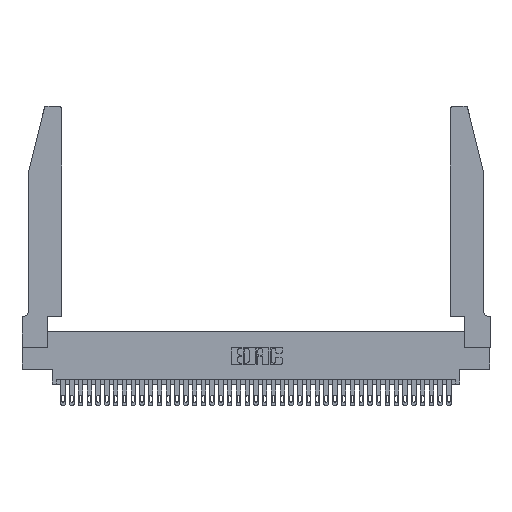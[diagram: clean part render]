
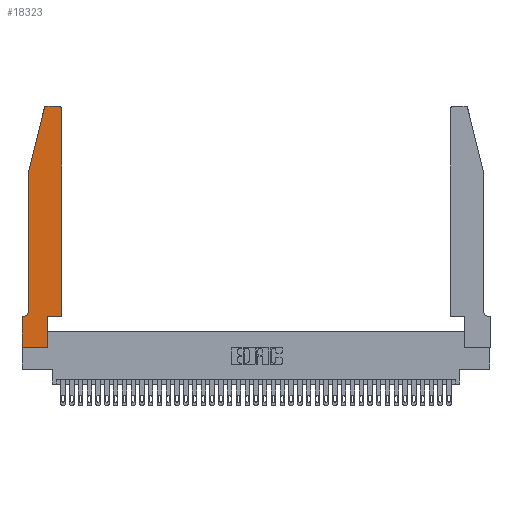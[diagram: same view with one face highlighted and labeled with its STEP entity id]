
A CAD part, top view. The second image highlights one B-rep face of the part: STEP entity #18323.
In plain terms, the highlighted planar face has unit normal (0, 0, 1).
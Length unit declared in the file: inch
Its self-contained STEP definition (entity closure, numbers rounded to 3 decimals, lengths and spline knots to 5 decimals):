
#86 = VERTEX_POINT ( 'NONE', #29668 ) ;
#151 = EDGE_CURVE ( 'NONE', #86, #35048, #34233, .T. ) ;
#384 = CARTESIAN_POINT ( 'NONE',  ( 0.0055, 0.42, 0.37 ) ) ;
#791 = ORIENTED_EDGE ( 'NONE', *, *, #26807, .T. ) ;
#1087 = EDGE_CURVE ( 'NONE', #15926, #29225, #2932, .T. ) ;
#1210 = ORIENTED_EDGE ( 'NONE', *, *, #21746, .T. ) ;
#1305 = DIRECTION ( 'NONE',  ( 1., 0., 0. ) ) ;
#2008 = CARTESIAN_POINT ( 'NONE',  ( 0.4505, 0.35, 0.37 ) ) ;
#2932 = LINE ( 'NONE', #17057, #21660 ) ;
#3139 = CARTESIAN_POINT ( 'NONE',  ( 0.2865, 0.35, 0.37 ) ) ;
#3264 = DIRECTION ( 'NONE',  ( 0., 1., 0. ) ) ;
#3406 = AXIS2_PLACEMENT_3D ( 'NONE', #35109, #4677, #38346 ) ;
#3493 = DIRECTION ( 'NONE',  ( 0., 0., -1. ) ) ;
#3570 = EDGE_CURVE ( 'NONE', #39554, #4459, #31378, .T. ) ;
#3728 = LINE ( 'NONE', #16018, #23432 ) ;
#3960 = ORIENTED_EDGE ( 'NONE', *, *, #21685, .T. ) ;
#4459 = VERTEX_POINT ( 'NONE', #37894 ) ;
#4586 = LINE ( 'NONE', #4966, #18542 ) ;
#4677 = DIRECTION ( 'NONE',  ( 0., 0., 1. ) ) ;
#4966 = CARTESIAN_POINT ( 'NONE',  ( 0., 0., 0.37 ) ) ;
#5246 = DIRECTION ( 'NONE',  ( -1., 0., 0. ) ) ;
#5284 = FACE_OUTER_BOUND ( 'NONE', #33183, .T. ) ;
#6537 = CARTESIAN_POINT ( 'NONE',  ( 0.0755, 0.42, 0.37 ) ) ;
#6699 = DIRECTION ( 'NONE',  ( 0., 1., 0. ) ) ;
#7874 = VERTEX_POINT ( 'NONE', #13865 ) ;
#8078 = VECTOR ( 'NONE', #21347, 39.37008 ) ;
#13363 = DIRECTION ( 'NONE',  ( 0., 0., 1. ) ) ;
#13376 = DIRECTION ( 'NONE',  ( 0., 0., 1. ) ) ;
#13865 = CARTESIAN_POINT ( 'NONE',  ( 0.4205, 2.75, 0.37 ) ) ;
#14188 = CARTESIAN_POINT ( 'NONE',  ( 0.2865, 0.35, 0.37 ) ) ;
#14258 = AXIS2_PLACEMENT_3D ( 'NONE', #34974, #13376, #38065 ) ;
#14449 = CARTESIAN_POINT ( 'NONE',  ( 0.4505, 2.72, 0.37 ) ) ;
#15034 = CARTESIAN_POINT ( 'NONE',  ( 0.0755, 2., 0.37 ) ) ;
#15319 = EDGE_CURVE ( 'NONE', #7874, #36643, #25417, .T. ) ;
#15326 = CARTESIAN_POINT ( 'NONE',  ( 0.0755, 2., 0.37 ) ) ;
#15926 = VERTEX_POINT ( 'NONE', #21176 ) ;
#16018 = CARTESIAN_POINT ( 'NONE',  ( 0.4505, 0.35, 0.37 ) ) ;
#16078 = VECTOR ( 'NONE', #27259, 39.37008 ) ;
#16306 = VECTOR ( 'NONE', #5246, 39.37008 ) ;
#16720 = ORIENTED_EDGE ( 'NONE', *, *, #38803, .T. ) ;
#17057 = CARTESIAN_POINT ( 'NONE',  ( 0., 0., 0.37 ) ) ;
#17156 = ORIENTED_EDGE ( 'NONE', *, *, #18286, .T. ) ;
#17606 = DIRECTION ( 'NONE',  ( -1., 0., 0. ) ) ;
#17999 = VERTEX_POINT ( 'NONE', #6537 ) ;
#18286 = EDGE_CURVE ( 'NONE', #36643, #86, #35721, .T. ) ;
#18323 = ADVANCED_FACE ( 'NONE', ( #5284 ), #22649, .T. ) ;
#18542 = VECTOR ( 'NONE', #22836, 39.37008 ) ;
#19097 = CARTESIAN_POINT ( 'NONE',  ( 0., 0.35, 0.37 ) ) ;
#19286 = AXIS2_PLACEMENT_3D ( 'NONE', #384, #3493, #24954 ) ;
#19828 = EDGE_CURVE ( 'NONE', #37520, #35860, #26470, .T. ) ;
#21176 = CARTESIAN_POINT ( 'NONE',  ( 0., 0., 0.37 ) ) ;
#21347 = DIRECTION ( 'NONE',  ( 0., -1., 0. ) ) ;
#21660 = VECTOR ( 'NONE', #22655, 39.37008 ) ;
#21685 = EDGE_CURVE ( 'NONE', #29225, #39554, #22448, .T. ) ;
#21746 = EDGE_CURVE ( 'NONE', #4459, #22698, #3728, .T. ) ;
#22448 = LINE ( 'NONE', #3139, #31055 ) ;
#22649 = PLANE ( 'NONE',  #14258 ) ;
#22655 = DIRECTION ( 'NONE',  ( 1., 0., 0. ) ) ;
#22698 = VERTEX_POINT ( 'NONE', #14449 ) ;
#22836 = DIRECTION ( 'NONE',  ( 0., -1., 0. ) ) ;
#23427 = ORIENTED_EDGE ( 'NONE', *, *, #34577, .T. ) ;
#23432 = VECTOR ( 'NONE', #6699, 39.37008 ) ;
#23865 = CARTESIAN_POINT ( 'NONE',  ( 0.284, 2.75, 0.37 ) ) ;
#24067 = ORIENTED_EDGE ( 'NONE', *, *, #151, .T. ) ;
#24617 = CARTESIAN_POINT ( 'NONE',  ( 0.0755, 2., 0.37 ) ) ;
#24731 = CIRCLE ( 'NONE', #19286, 0.07 ) ;
#24954 = DIRECTION ( 'NONE',  ( -1., 0., 0. ) ) ;
#25327 = CARTESIAN_POINT ( 'NONE',  ( 0.4205, 2.72, 0.37 ) ) ;
#25417 = LINE ( 'NONE', #39052, #16306 ) ;
#25946 = ORIENTED_EDGE ( 'NONE', *, *, #15319, .T. ) ;
#26470 = LINE ( 'NONE', #27243, #33675 ) ;
#26807 = EDGE_CURVE ( 'NONE', #17999, #37520, #24731, .T. ) ;
#27243 = CARTESIAN_POINT ( 'NONE',  ( 0.0755, 0.35, 0.37 ) ) ;
#27259 = DIRECTION ( 'NONE',  ( 1., 0., 0. ) ) ;
#27639 = ORIENTED_EDGE ( 'NONE', *, *, #3570, .T. ) ;
#28636 = ORIENTED_EDGE ( 'NONE', *, *, #19828, .T. ) ;
#29003 = CARTESIAN_POINT ( 'NONE',  ( 0.0055, 0.35, 0.37 ) ) ;
#29225 = VERTEX_POINT ( 'NONE', #30435 ) ;
#29668 = CARTESIAN_POINT ( 'NONE',  ( 0.25487, 2.72718, 0.37 ) ) ;
#30379 = VECTOR ( 'NONE', #36661, 39.37008 ) ;
#30435 = CARTESIAN_POINT ( 'NONE',  ( 0.2865, 0., 0.37 ) ) ;
#31055 = VECTOR ( 'NONE', #3264, 39.37008 ) ;
#31378 = LINE ( 'NONE', #2008, #16078 ) ;
#31444 = ORIENTED_EDGE ( 'NONE', *, *, #1087, .T. ) ;
#32316 = EDGE_CURVE ( 'NONE', #35048, #17999, #33091, .T. ) ;
#33091 = LINE ( 'NONE', #15034, #8078 ) ;
#33183 = EDGE_LOOP ( 'NONE', ( #25946, #17156, #24067, #33551, #791, #28636, #16720, #31444, #3960, #27639, #1210, #23427 ) ) ;
#33551 = ORIENTED_EDGE ( 'NONE', *, *, #32316, .T. ) ;
#33675 = VECTOR ( 'NONE', #17606, 39.37008 ) ;
#34233 = LINE ( 'NONE', #15326, #30379 ) ;
#34577 = EDGE_CURVE ( 'NONE', #22698, #7874, #38686, .T. ) ;
#34974 = CARTESIAN_POINT ( 'NONE',  ( 0., 0.35, 0.37 ) ) ;
#35048 = VERTEX_POINT ( 'NONE', #24617 ) ;
#35109 = CARTESIAN_POINT ( 'NONE',  ( 0.284, 2.72, 0.37 ) ) ;
#35721 = CIRCLE ( 'NONE', #3406, 0.03 ) ;
#35860 = VERTEX_POINT ( 'NONE', #19097 ) ;
#36643 = VERTEX_POINT ( 'NONE', #23865 ) ;
#36661 = DIRECTION ( 'NONE',  ( -0.239, -0.971, 0. ) ) ;
#37330 = AXIS2_PLACEMENT_3D ( 'NONE', #25327, #13363, #1305 ) ;
#37520 = VERTEX_POINT ( 'NONE', #29003 ) ;
#37894 = CARTESIAN_POINT ( 'NONE',  ( 0.4505, 0.35, 0.37 ) ) ;
#38065 = DIRECTION ( 'NONE',  ( 1., 0., 0. ) ) ;
#38346 = DIRECTION ( 'NONE',  ( 1., 0., 0. ) ) ;
#38686 = CIRCLE ( 'NONE', #37330, 0.03 ) ;
#38803 = EDGE_CURVE ( 'NONE', #35860, #15926, #4586, .T. ) ;
#39052 = CARTESIAN_POINT ( 'NONE',  ( 0.2605, 2.75, 0.37 ) ) ;
#39554 = VERTEX_POINT ( 'NONE', #14188 ) ;
